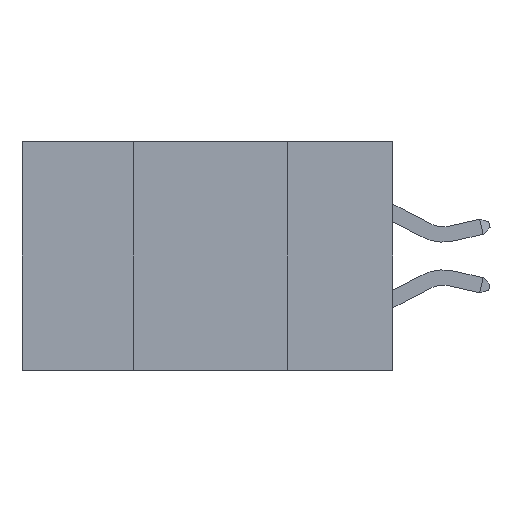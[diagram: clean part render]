
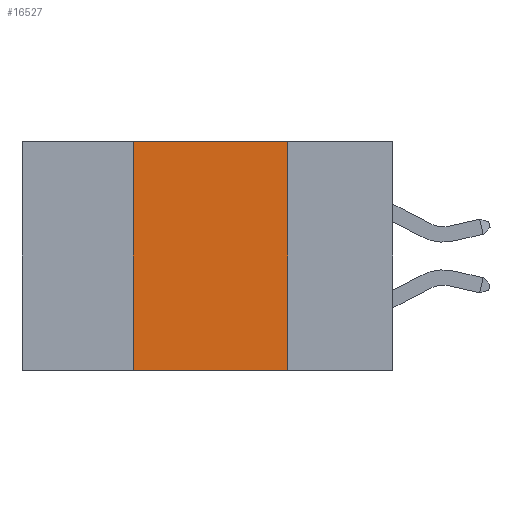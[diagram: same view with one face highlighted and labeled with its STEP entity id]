
A CAD part, left-side view. The second image highlights one B-rep face of the part: STEP entity #16527.
In plain terms, the highlighted planar face has unit normal (-1, 0, 0).
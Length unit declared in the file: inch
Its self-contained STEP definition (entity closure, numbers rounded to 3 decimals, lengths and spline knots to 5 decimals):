
#1052 = CARTESIAN_POINT ( 'NONE',  ( 0., 0.6, 0. ) ) ;
#1442 = VECTOR ( 'NONE', #17716, 39.37008 ) ;
#1883 = LINE ( 'NONE', #13398, #1442 ) ;
#1959 = PLANE ( 'NONE',  #7674 ) ;
#2226 = VERTEX_POINT ( 'NONE', #6451 ) ;
#2349 = CARTESIAN_POINT ( 'NONE',  ( 0., 0.17, 0. ) ) ;
#2447 = EDGE_CURVE ( 'NONE', #7936, #8204, #16555, .T. ) ;
#2896 = VERTEX_POINT ( 'NONE', #2349 ) ;
#3502 = VECTOR ( 'NONE', #17133, 39.37008 ) ;
#4875 = VECTOR ( 'NONE', #12749, 39.37008 ) ;
#5995 = CARTESIAN_POINT ( 'NONE',  ( 0., 0.42, -0.37 ) ) ;
#6363 = LINE ( 'NONE', #11649, #3502 ) ;
#6451 = CARTESIAN_POINT ( 'NONE',  ( 0., 0.17, -0.37 ) ) ;
#7148 = EDGE_CURVE ( 'NONE', #7936, #2226, #6363, .T. ) ;
#7179 = ORIENTED_EDGE ( 'NONE', *, *, #14360, .F. ) ;
#7590 = ORIENTED_EDGE ( 'NONE', *, *, #7148, .T. ) ;
#7674 = AXIS2_PLACEMENT_3D ( 'NONE', #17612, #8938, #10339 ) ;
#7936 = VERTEX_POINT ( 'NONE', #5995 ) ;
#8204 = VERTEX_POINT ( 'NONE', #11027 ) ;
#8227 = FACE_OUTER_BOUND ( 'NONE', #14028, .T. ) ;
#8938 = DIRECTION ( 'NONE',  ( 1., 0., 0. ) ) ;
#9386 = EDGE_CURVE ( 'NONE', #2896, #2226, #1883, .T. ) ;
#10339 = DIRECTION ( 'NONE',  ( 0., 0., -1. ) ) ;
#11027 = CARTESIAN_POINT ( 'NONE',  ( 0., 0.42, 0. ) ) ;
#11649 = CARTESIAN_POINT ( 'NONE',  ( 0., 0.6, -0.37 ) ) ;
#12749 = DIRECTION ( 'NONE',  ( 0., 0., 1. ) ) ;
#13001 = ORIENTED_EDGE ( 'NONE', *, *, #9386, .F. ) ;
#13398 = CARTESIAN_POINT ( 'NONE',  ( 0., 0.17, 0. ) ) ;
#14028 = EDGE_LOOP ( 'NONE', ( #13001, #7179, #17485, #7590 ) ) ;
#14244 = LINE ( 'NONE', #1052, #17320 ) ;
#14360 = EDGE_CURVE ( 'NONE', #8204, #2896, #14244, .T. ) ;
#15307 = CARTESIAN_POINT ( 'NONE',  ( 0., 0.42, 0. ) ) ;
#16527 = ADVANCED_FACE ( 'NONE', ( #8227 ), #1959, .F. ) ;
#16555 = LINE ( 'NONE', #15307, #4875 ) ;
#16631 = DIRECTION ( 'NONE',  ( 0., -1., 0. ) ) ;
#17133 = DIRECTION ( 'NONE',  ( 0., -1., 0. ) ) ;
#17320 = VECTOR ( 'NONE', #16631, 39.37008 ) ;
#17485 = ORIENTED_EDGE ( 'NONE', *, *, #2447, .F. ) ;
#17612 = CARTESIAN_POINT ( 'NONE',  ( 0., 0.6, 0. ) ) ;
#17716 = DIRECTION ( 'NONE',  ( 0., 0., -1. ) ) ;
